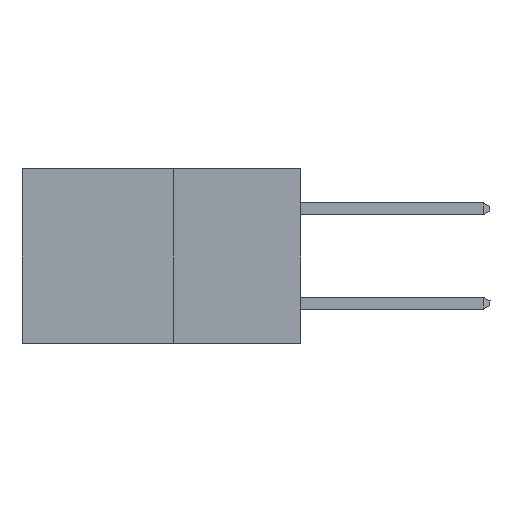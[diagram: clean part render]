
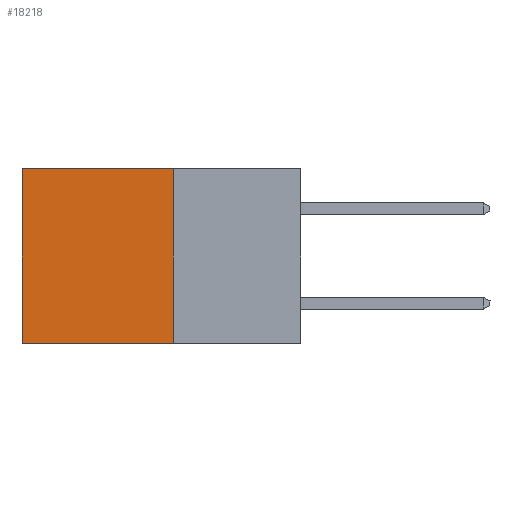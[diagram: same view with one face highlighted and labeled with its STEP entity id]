
A CAD part, left-side view. The second image highlights one B-rep face of the part: STEP entity #18218.
In plain terms, the highlighted planar face has unit normal (-1, 0, 0).
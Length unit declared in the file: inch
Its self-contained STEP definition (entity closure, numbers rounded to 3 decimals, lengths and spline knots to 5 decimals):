
#346 = CARTESIAN_POINT ( 'NONE',  ( 0.277, 0.27, 0. ) ) ;
#671 = VECTOR ( 'NONE', #29874, 39.37008 ) ;
#958 = AXIS2_PLACEMENT_3D ( 'NONE', #15376, #1136, #17680 ) ;
#1136 = DIRECTION ( 'NONE',  ( 1., 0., 0. ) ) ;
#1398 = CARTESIAN_POINT ( 'NONE',  ( 0.277, 0.27, -0.37 ) ) ;
#2938 = VECTOR ( 'NONE', #26583, 39.37008 ) ;
#3429 = EDGE_CURVE ( 'NONE', #22540, #16643, #18036, .T. ) ;
#3657 = LINE ( 'NONE', #15235, #2938 ) ;
#4825 = DIRECTION ( 'NONE',  ( 0., 0., -1. ) ) ;
#4855 = VERTEX_POINT ( 'NONE', #1398 ) ;
#5039 = EDGE_CURVE ( 'NONE', #16643, #22186, #29261, .T. ) ;
#5119 = DIRECTION ( 'NONE',  ( 0., 1., 0. ) ) ;
#6090 = ORIENTED_EDGE ( 'NONE', *, *, #5039, .T. ) ;
#6990 = LINE ( 'NONE', #25262, #671 ) ;
#7389 = EDGE_LOOP ( 'NONE', ( #6090, #18047, #14299, #10711 ) ) ;
#10711 = ORIENTED_EDGE ( 'NONE', *, *, #3429, .T. ) ;
#11840 = VECTOR ( 'NONE', #5119, 39.37008 ) ;
#14299 = ORIENTED_EDGE ( 'NONE', *, *, #18932, .F. ) ;
#15235 = CARTESIAN_POINT ( 'NONE',  ( 0.277, 0.27, -0.37 ) ) ;
#15376 = CARTESIAN_POINT ( 'NONE',  ( 0.277, 0.27, -0.37 ) ) ;
#16405 = VECTOR ( 'NONE', #4825, 39.37008 ) ;
#16632 = CARTESIAN_POINT ( 'NONE',  ( 0.277, 0.59, -0.37 ) ) ;
#16643 = VERTEX_POINT ( 'NONE', #19711 ) ;
#17680 = DIRECTION ( 'NONE',  ( 0., 0., -1. ) ) ;
#18036 = LINE ( 'NONE', #346, #11840 ) ;
#18047 = ORIENTED_EDGE ( 'NONE', *, *, #19874, .F. ) ;
#18218 = ADVANCED_FACE ( 'NONE', ( #22801 ), #29049, .F. ) ;
#18932 = EDGE_CURVE ( 'NONE', #22540, #4855, #3657, .T. ) ;
#19711 = CARTESIAN_POINT ( 'NONE',  ( 0.277, 0.59, 0. ) ) ;
#19874 = EDGE_CURVE ( 'NONE', #4855, #22186, #6990, .T. ) ;
#21553 = CARTESIAN_POINT ( 'NONE',  ( 0.277, 0.27, 0. ) ) ;
#22186 = VERTEX_POINT ( 'NONE', #29429 ) ;
#22540 = VERTEX_POINT ( 'NONE', #21553 ) ;
#22801 = FACE_OUTER_BOUND ( 'NONE', #7389, .T. ) ;
#25262 = CARTESIAN_POINT ( 'NONE',  ( 0.277, 0.27, -0.37 ) ) ;
#26583 = DIRECTION ( 'NONE',  ( 0., 0., -1. ) ) ;
#29049 = PLANE ( 'NONE',  #958 ) ;
#29261 = LINE ( 'NONE', #16632, #16405 ) ;
#29429 = CARTESIAN_POINT ( 'NONE',  ( 0.277, 0.59, -0.37 ) ) ;
#29874 = DIRECTION ( 'NONE',  ( 0., 1., 0. ) ) ;
